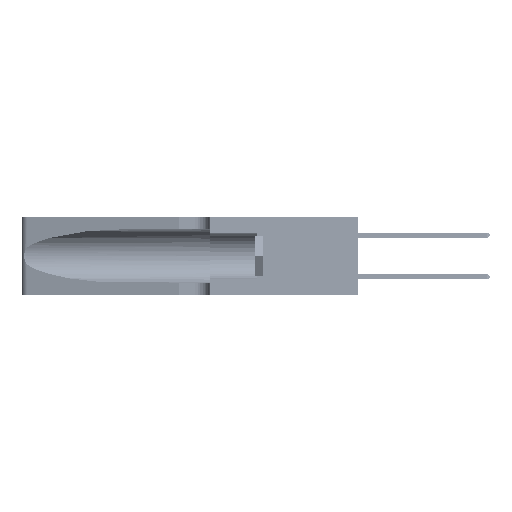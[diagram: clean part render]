
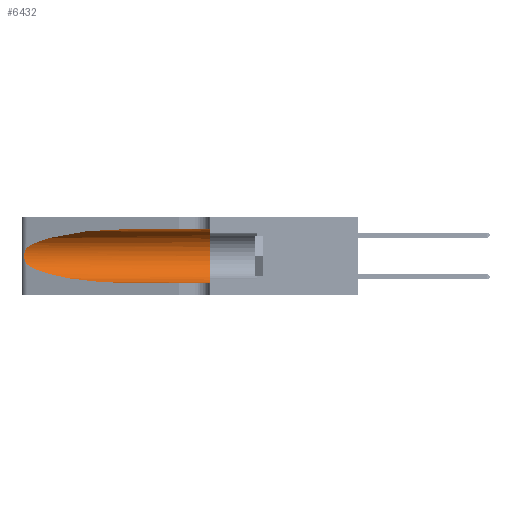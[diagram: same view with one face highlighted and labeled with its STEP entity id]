
A CAD part, left-side view. The second image highlights one B-rep face of the part: STEP entity #6432.
In plain terms, the highlighted cylindrical face has radius 3.308 mm (diameter 6.617 mm), a partial arc.
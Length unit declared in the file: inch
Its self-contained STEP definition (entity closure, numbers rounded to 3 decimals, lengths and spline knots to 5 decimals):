
#746 = CARTESIAN_POINT ( 'NONE',  ( 0.25487, 1.22718, 0.22369 ) ) ;
#1116 = VERTEX_POINT ( 'NONE', #1511 ) ;
#1511 = CARTESIAN_POINT ( 'NONE',  ( 0.1305, 0.35, 0.05475 ) ) ;
#1873 = CARTESIAN_POINT ( 'NONE',  ( 0.25639, 1.23184, 0.21858 ) ) ;
#2594 = CYLINDRICAL_SURFACE ( 'NONE', #4079, 0.13025 ) ;
#2895 = VECTOR ( 'NONE', #39174, 39.37008 ) ;
#3922 = CARTESIAN_POINT ( 'NONE',  ( 0.18966, 0.96281, 0.05475 ) ) ;
#4079 = AXIS2_PLACEMENT_3D ( 'NONE', #5285, #13684, #34310 ) ;
#5151 = CARTESIAN_POINT ( 'NONE',  ( 0.25487, 1.22718, 0.14631 ) ) ;
#5285 = CARTESIAN_POINT ( 'NONE',  ( 0.1305, 1.61858, 0.185 ) ) ;
#5524 = CARTESIAN_POINT ( 'NONE',  ( 0.26018, 1.23835, 0.19895 ) ) ;
#5868 = CARTESIAN_POINT ( 'NONE',  ( 0.26075, 1.23896, 0.19203 ) ) ;
#6432 = ADVANCED_FACE ( 'NONE', ( #32581 ), #2594, .F. ) ;
#6718 = VERTEX_POINT ( 'NONE', #15119 ) ;
#7616 = LINE ( 'NONE', #20887, #47525 ) ;
#8108 = CARTESIAN_POINT ( 'NONE',  ( 0.2373, 1.15595, 0.08982 ) ) ;
#8235 = DIRECTION ( 'NONE',  ( 0., -1., 0. ) ) ;
#8694 = VERTEX_POINT ( 'NONE', #36682 ) ;
#8952 = CARTESIAN_POINT ( 'NONE',  ( 0.18966, 0.96281, 0.31525 ) ) ;
#10114 = CARTESIAN_POINT ( 'NONE',  ( 0.1305, 1.61858, 0.05475 ) ) ;
#10928 = B_SPLINE_CURVE_WITH_KNOTS ( 'NONE', 3,
 ( #34921, #18497, #1873, #22165, #17744, #5524, #5868, #43144, #18318, #39138, #43326, #43511, #51924, #5151 ),
 .UNSPECIFIED., .F., .F.,
 ( 4, 2, 2, 2, 2, 2, 4 ),
 ( 0., 0.00027, 0.00053, 0.00107, 0.0016, 0.00187, 0.00214 ),
 .UNSPECIFIED. ) ;
#12322 = CARTESIAN_POINT ( 'NONE',  ( 0.1305, 0.72297, 0.05475 ) ) ;
#12926 = AXIS2_PLACEMENT_3D ( 'NONE', #25205, #50048, #24827 ) ;
#13406 = ORIENTED_EDGE ( 'NONE', *, *, #48365, .F. ) ;
#13684 = DIRECTION ( 'NONE',  ( 0., -1., 0. ) ) ;
#13705 = CARTESIAN_POINT ( 'NONE',  ( 0.1305, 0.72297, 0.31525 ) ) ;
#15119 = CARTESIAN_POINT ( 'NONE',  ( 0.1305, 0.35, 0.31525 ) ) ;
#15441 = CARTESIAN_POINT ( 'NONE',  ( 0.1305, 0.72297, 0.05475 ) ) ;
#17744 = CARTESIAN_POINT ( 'NONE',  ( 0.25854, 1.2359, 0.20912 ) ) ;
#17745 = VERTEX_POINT ( 'NONE', #44111 ) ;
#17906 = CARTESIAN_POINT ( 'NONE',  ( 0.2373, 1.15595, 0.28018 ) ) ;
#18318 = CARTESIAN_POINT ( 'NONE',  ( 0.26017, 1.23833, 0.17102 ) ) ;
#18497 = CARTESIAN_POINT ( 'NONE',  ( 0.25555, 1.22994, 0.2215 ) ) ;
#20887 = CARTESIAN_POINT ( 'NONE',  ( 0.1305, 1.61858, 0.31525 ) ) ;
#20928 = VERTEX_POINT ( 'NONE', #15441 ) ;
#21177 = CIRCLE ( 'NONE', #12926, 0.13025 ) ;
#22165 = CARTESIAN_POINT ( 'NONE',  ( 0.25787, 1.23484, 0.2124 ) ) ;
#23905 = ORIENTED_EDGE ( 'NONE', *, *, #30441, .T. ) ;
#24038 = EDGE_CURVE ( 'NONE', #33331, #17745, #10928, .T. ) ;
#24231 = CARTESIAN_POINT ( 'NONE',  ( 0.25487, 1.22718, 0.22369 ) ) ;
#24827 = DIRECTION ( 'NONE',  ( 0., 0., 1. ) ) ;
#25205 = CARTESIAN_POINT ( 'NONE',  ( 0.1305, 0.35, 0.185 ) ) ;
#30441 = EDGE_CURVE ( 'NONE', #20928, #1116, #49266, .T. ) ;
#32581 = FACE_OUTER_BOUND ( 'NONE', #43576, .T. ) ;
#33331 = VERTEX_POINT ( 'NONE', #24231 ) ;
#34310 = DIRECTION ( 'NONE',  ( 0., 0., -1. ) ) ;
#34347 =( BOUNDED_CURVE ( )  B_SPLINE_CURVE ( 3, ( #13705, #8952, #17906, #746 ),
 .UNSPECIFIED., .F., .F. ) 
 B_SPLINE_CURVE_WITH_KNOTS ( ( 4, 4 ),
 ( 1.5708, 2.84003 ),
 .UNSPECIFIED. ) 
 CURVE ( )  GEOMETRIC_REPRESENTATION_ITEM ( )  RATIONAL_B_SPLINE_CURVE ( ( 1., 0.87, 0.87, 1. ) ) 
 REPRESENTATION_ITEM ( '' )  );
#34921 = CARTESIAN_POINT ( 'NONE',  ( 0.25487, 1.22718, 0.22369 ) ) ;
#35589 = EDGE_CURVE ( 'NONE', #17745, #20928, #49771, .T. ) ;
#36682 = CARTESIAN_POINT ( 'NONE',  ( 0.1305, 0.72297, 0.31525 ) ) ;
#37124 = ORIENTED_EDGE ( 'NONE', *, *, #35589, .T. ) ;
#37344 = CARTESIAN_POINT ( 'NONE',  ( 0.25487, 1.22718, 0.14631 ) ) ;
#39138 = CARTESIAN_POINT ( 'NONE',  ( 0.25856, 1.23593, 0.16098 ) ) ;
#39171 = EDGE_CURVE ( 'NONE', #6718, #1116, #21177, .T. ) ;
#39174 = DIRECTION ( 'NONE',  ( 0., -1., 0. ) ) ;
#40589 = EDGE_CURVE ( 'NONE', #8694, #33331, #34347, .T. ) ;
#43144 = CARTESIAN_POINT ( 'NONE',  ( 0.26075, 1.23896, 0.178 ) ) ;
#43326 = CARTESIAN_POINT ( 'NONE',  ( 0.25789, 1.23486, 0.15765 ) ) ;
#43511 = CARTESIAN_POINT ( 'NONE',  ( 0.25639, 1.23186, 0.15144 ) ) ;
#43576 = EDGE_LOOP ( 'NONE', ( #44929, #52292, #37124, #23905, #43869, #13406 ) ) ;
#43869 = ORIENTED_EDGE ( 'NONE', *, *, #39171, .F. ) ;
#44111 = CARTESIAN_POINT ( 'NONE',  ( 0.25487, 1.22718, 0.14631 ) ) ;
#44929 = ORIENTED_EDGE ( 'NONE', *, *, #40589, .T. ) ;
#47525 = VECTOR ( 'NONE', #8235, 39.37008 ) ;
#48365 = EDGE_CURVE ( 'NONE', #8694, #6718, #7616, .T. ) ;
#49266 = LINE ( 'NONE', #10114, #2895 ) ;
#49771 =( BOUNDED_CURVE ( )  B_SPLINE_CURVE ( 3, ( #37344, #8108, #3922, #12322 ),
 .UNSPECIFIED., .F., .T. ) 
 B_SPLINE_CURVE_WITH_KNOTS ( ( 4, 4 ),
 ( 3.44316, 4.71239 ),
 .UNSPECIFIED. ) 
 CURVE ( )  GEOMETRIC_REPRESENTATION_ITEM ( )  RATIONAL_B_SPLINE_CURVE ( ( 1., 0.87, 0.87, 1. ) ) 
 REPRESENTATION_ITEM ( '' )  );
#50048 = DIRECTION ( 'NONE',  ( 0., 1., 0. ) ) ;
#51924 = CARTESIAN_POINT ( 'NONE',  ( 0.25555, 1.22993, 0.14849 ) ) ;
#52292 = ORIENTED_EDGE ( 'NONE', *, *, #24038, .T. ) ;
